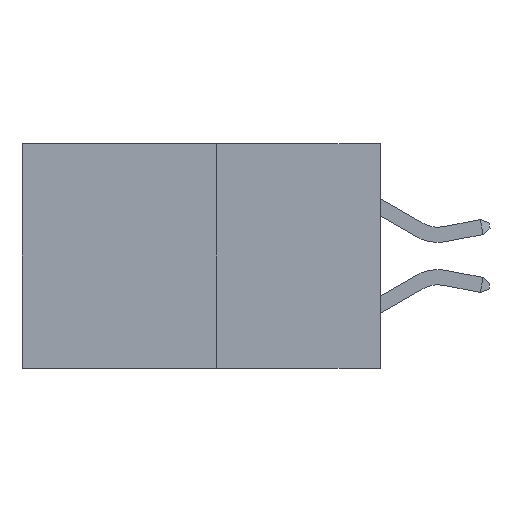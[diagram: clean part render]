
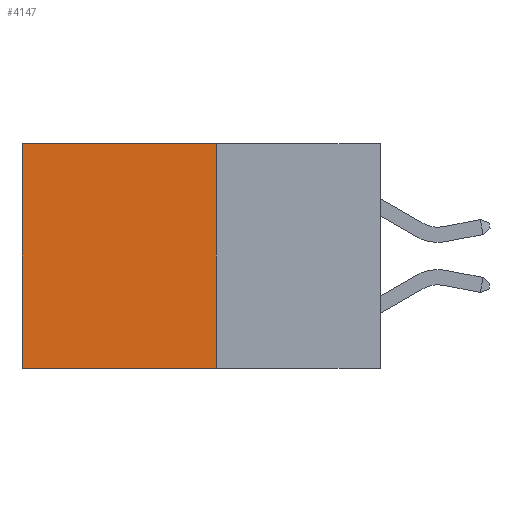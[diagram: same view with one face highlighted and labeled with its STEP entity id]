
A CAD part, left-side view. The second image highlights one B-rep face of the part: STEP entity #4147.
In plain terms, the highlighted planar face has unit normal (-1, 0, 0).
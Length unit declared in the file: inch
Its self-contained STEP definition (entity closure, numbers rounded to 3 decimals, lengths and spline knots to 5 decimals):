
#485 = VECTOR ( 'NONE', #10612, 39.37008 ) ;
#600 = VECTOR ( 'NONE', #6687, 39.37008 ) ;
#1428 = VECTOR ( 'NONE', #7274, 39.37008 ) ;
#1433 = VERTEX_POINT ( 'NONE', #3189 ) ;
#2721 = LINE ( 'NONE', #3013, #4844 ) ;
#2879 = LINE ( 'NONE', #8988, #485 ) ;
#3013 = CARTESIAN_POINT ( 'NONE',  ( 0.277, 0.27, -0.37 ) ) ;
#3189 = CARTESIAN_POINT ( 'NONE',  ( 0.277, 0.27, 0. ) ) ;
#3269 = EDGE_CURVE ( 'NONE', #8237, #5788, #5993, .T. ) ;
#3319 = EDGE_CURVE ( 'NONE', #1433, #10814, #2721, .T. ) ;
#3403 = EDGE_LOOP ( 'NONE', ( #10692, #10615, #10702, #10689 ) ) ;
#3622 = FACE_OUTER_BOUND ( 'NONE', #3403, .T. ) ;
#3726 = LINE ( 'NONE', #7088, #1428 ) ;
#4147 = ADVANCED_FACE ( 'NONE', ( #3622 ), #7593, .F. ) ;
#4844 = VECTOR ( 'NONE', #6164, 39.37008 ) ;
#5356 = CARTESIAN_POINT ( 'NONE',  ( 0.277, 0.27, -0.37 ) ) ;
#5788 = VERTEX_POINT ( 'NONE', #6017 ) ;
#5993 = LINE ( 'NONE', #11331, #600 ) ;
#6017 = CARTESIAN_POINT ( 'NONE',  ( 0.277, 0.59, -0.37 ) ) ;
#6164 = DIRECTION ( 'NONE',  ( 0., 0., -1. ) ) ;
#6497 = EDGE_CURVE ( 'NONE', #10814, #5788, #3726, .T. ) ;
#6687 = DIRECTION ( 'NONE',  ( 0., 0., -1. ) ) ;
#7088 = CARTESIAN_POINT ( 'NONE',  ( 0.277, 0.27, -0.37 ) ) ;
#7198 = DIRECTION ( 'NONE',  ( 0., 0., -1. ) ) ;
#7272 = DIRECTION ( 'NONE',  ( 1., 0., 0. ) ) ;
#7274 = DIRECTION ( 'NONE',  ( 0., 1., 0. ) ) ;
#7387 = CARTESIAN_POINT ( 'NONE',  ( 0.277, 0.27, -0.37 ) ) ;
#7593 = PLANE ( 'NONE',  #11144 ) ;
#8237 = VERTEX_POINT ( 'NONE', #9747 ) ;
#8262 = EDGE_CURVE ( 'NONE', #1433, #8237, #2879, .T. ) ;
#8988 = CARTESIAN_POINT ( 'NONE',  ( 0.277, 0.27, 0. ) ) ;
#9747 = CARTESIAN_POINT ( 'NONE',  ( 0.277, 0.59, 0. ) ) ;
#10612 = DIRECTION ( 'NONE',  ( 0., 1., 0. ) ) ;
#10615 = ORIENTED_EDGE ( 'NONE', *, *, #6497, .F. ) ;
#10689 = ORIENTED_EDGE ( 'NONE', *, *, #8262, .T. ) ;
#10692 = ORIENTED_EDGE ( 'NONE', *, *, #3269, .T. ) ;
#10702 = ORIENTED_EDGE ( 'NONE', *, *, #3319, .F. ) ;
#10814 = VERTEX_POINT ( 'NONE', #5356 ) ;
#11144 = AXIS2_PLACEMENT_3D ( 'NONE', #7387, #7272, #7198 ) ;
#11331 = CARTESIAN_POINT ( 'NONE',  ( 0.277, 0.59, -0.37 ) ) ;
